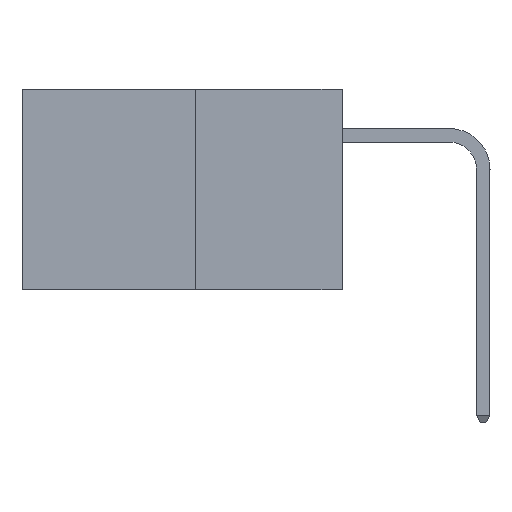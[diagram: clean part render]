
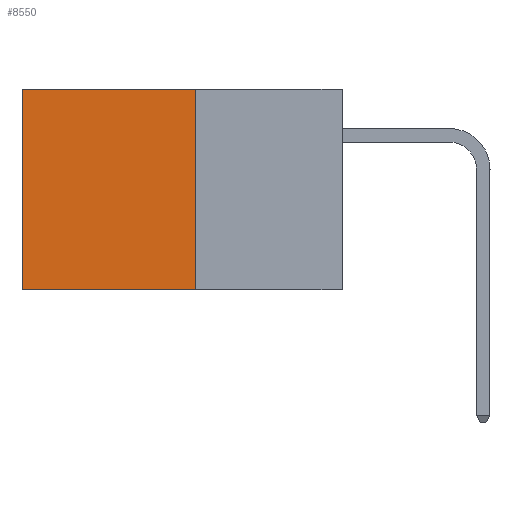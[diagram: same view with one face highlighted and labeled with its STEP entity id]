
A CAD part, left-side view. The second image highlights one B-rep face of the part: STEP entity #8550.
In plain terms, the highlighted planar face has unit normal (-1, 0, 0).
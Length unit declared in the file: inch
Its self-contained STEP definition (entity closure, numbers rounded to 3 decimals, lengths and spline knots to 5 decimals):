
#122 = VERTEX_POINT ( 'NONE', #5549 ) ;
#212 = FACE_OUTER_BOUND ( 'NONE', #2996, .T. ) ;
#271 = VECTOR ( 'NONE', #2479, 39.37008 ) ;
#458 = CARTESIAN_POINT ( 'NONE',  ( 0.277, 0.27, 0. ) ) ;
#596 = EDGE_CURVE ( 'NONE', #743, #8906, #12375, .T. ) ;
#743 = VERTEX_POINT ( 'NONE', #10704 ) ;
#1456 = EDGE_CURVE ( 'NONE', #10115, #743, #10000, .T. ) ;
#1821 = ORIENTED_EDGE ( 'NONE', *, *, #2721, .T. ) ;
#1833 = DIRECTION ( 'NONE',  ( 1., 0., 0. ) ) ;
#2361 = VECTOR ( 'NONE', #8571, 39.37008 ) ;
#2479 = DIRECTION ( 'NONE',  ( 0., 1., 0. ) ) ;
#2721 = EDGE_CURVE ( 'NONE', #10115, #122, #3536, .T. ) ;
#2996 = EDGE_LOOP ( 'NONE', ( #10310, #3576, #6343, #1821 ) ) ;
#3243 = VECTOR ( 'NONE', #5316, 39.37008 ) ;
#3401 = CARTESIAN_POINT ( 'NONE',  ( 0.277, 0.59, -0.37 ) ) ;
#3536 = LINE ( 'NONE', #10084, #3243 ) ;
#3576 = ORIENTED_EDGE ( 'NONE', *, *, #596, .F. ) ;
#5316 = DIRECTION ( 'NONE',  ( 0., 1., 0. ) ) ;
#5549 = CARTESIAN_POINT ( 'NONE',  ( 0.277, 0.59, 0. ) ) ;
#5657 = PLANE ( 'NONE',  #10233 ) ;
#6343 = ORIENTED_EDGE ( 'NONE', *, *, #1456, .F. ) ;
#6814 = VECTOR ( 'NONE', #10088, 39.37008 ) ;
#7577 = CARTESIAN_POINT ( 'NONE',  ( 0.277, 0.27, -0.37 ) ) ;
#7735 = EDGE_CURVE ( 'NONE', #122, #8906, #11593, .T. ) ;
#8053 = CARTESIAN_POINT ( 'NONE',  ( 0.277, 0.59, -0.37 ) ) ;
#8538 = DIRECTION ( 'NONE',  ( 0., 0., -1. ) ) ;
#8550 = ADVANCED_FACE ( 'NONE', ( #212 ), #5657, .F. ) ;
#8571 = DIRECTION ( 'NONE',  ( 0., 0., -1. ) ) ;
#8906 = VERTEX_POINT ( 'NONE', #8053 ) ;
#9533 = CARTESIAN_POINT ( 'NONE',  ( 0.277, 0.27, -0.37 ) ) ;
#10000 = LINE ( 'NONE', #9533, #2361 ) ;
#10084 = CARTESIAN_POINT ( 'NONE',  ( 0.277, 0.27, 0. ) ) ;
#10088 = DIRECTION ( 'NONE',  ( 0., 0., -1. ) ) ;
#10115 = VERTEX_POINT ( 'NONE', #458 ) ;
#10233 = AXIS2_PLACEMENT_3D ( 'NONE', #7577, #1833, #8538 ) ;
#10310 = ORIENTED_EDGE ( 'NONE', *, *, #7735, .T. ) ;
#10437 = CARTESIAN_POINT ( 'NONE',  ( 0.277, 0.27, -0.37 ) ) ;
#10704 = CARTESIAN_POINT ( 'NONE',  ( 0.277, 0.27, -0.37 ) ) ;
#11593 = LINE ( 'NONE', #3401, #6814 ) ;
#12375 = LINE ( 'NONE', #10437, #271 ) ;
